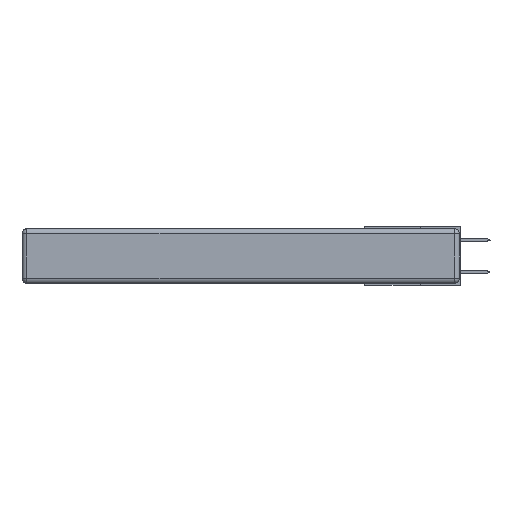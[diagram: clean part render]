
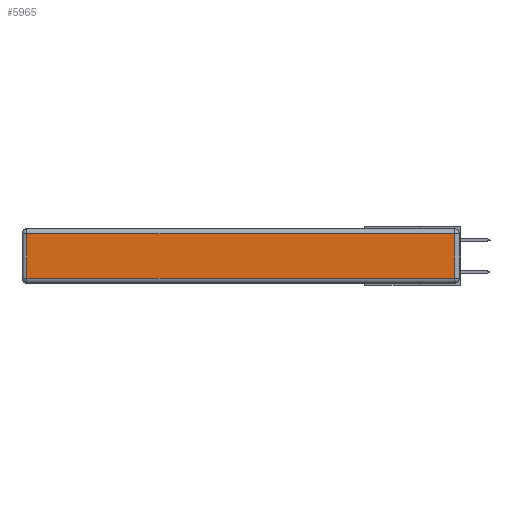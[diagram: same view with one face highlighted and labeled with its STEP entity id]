
A CAD part, left-side view. The second image highlights one B-rep face of the part: STEP entity #5965.
In plain terms, the highlighted planar face has unit normal (-1, 0, 0).
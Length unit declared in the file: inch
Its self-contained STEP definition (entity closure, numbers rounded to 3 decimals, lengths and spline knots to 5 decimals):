
#509 = VECTOR ( 'NONE', #15743, 39.37008 ) ;
#979 = EDGE_LOOP ( 'NONE', ( #4336, #14301, #8746, #16930 ) ) ;
#1898 = CARTESIAN_POINT ( 'NONE',  ( 0., 2.72, -0.03 ) ) ;
#4126 = AXIS2_PLACEMENT_3D ( 'NONE', #28150, #23586, #25646 ) ;
#4127 = EDGE_CURVE ( 'NONE', #7044, #15116, #28561, .T. ) ;
#4336 = ORIENTED_EDGE ( 'NONE', *, *, #13234, .T. ) ;
#5965 = ADVANCED_FACE ( 'NONE', ( #17543 ), #16148, .T. ) ;
#6725 = CARTESIAN_POINT ( 'NONE',  ( 0., 0.03, -0.313 ) ) ;
#7044 = VERTEX_POINT ( 'NONE', #15593 ) ;
#8746 = ORIENTED_EDGE ( 'NONE', *, *, #4127, .T. ) ;
#9346 = EDGE_CURVE ( 'NONE', #16502, #7044, #11460, .T. ) ;
#9361 = DIRECTION ( 'NONE',  ( 0., 0., -1. ) ) ;
#9627 = DIRECTION ( 'NONE',  ( 0., 0., 1. ) ) ;
#11460 = LINE ( 'NONE', #24569, #31768 ) ;
#13234 = EDGE_CURVE ( 'NONE', #30001, #16502, #29903, .T. ) ;
#14301 = ORIENTED_EDGE ( 'NONE', *, *, #9346, .T. ) ;
#15116 = VERTEX_POINT ( 'NONE', #1898 ) ;
#15593 = CARTESIAN_POINT ( 'NONE',  ( 0., 0.03, -0.03 ) ) ;
#15743 = DIRECTION ( 'NONE',  ( 0., 1., 0. ) ) ;
#15960 = CARTESIAN_POINT ( 'NONE',  ( 0., 2.75, -0.03 ) ) ;
#16148 = PLANE ( 'NONE',  #4126 ) ;
#16502 = VERTEX_POINT ( 'NONE', #6725 ) ;
#16624 = VECTOR ( 'NONE', #17464, 39.37008 ) ;
#16930 = ORIENTED_EDGE ( 'NONE', *, *, #19333, .T. ) ;
#17464 = DIRECTION ( 'NONE',  ( 0., -1., 0. ) ) ;
#17543 = FACE_OUTER_BOUND ( 'NONE', #979, .T. ) ;
#19012 = LINE ( 'NONE', #27121, #22499 ) ;
#19333 = EDGE_CURVE ( 'NONE', #15116, #30001, #19012, .T. ) ;
#22499 = VECTOR ( 'NONE', #9361, 39.37008 ) ;
#22830 = CARTESIAN_POINT ( 'NONE',  ( 0., 0., -0.313 ) ) ;
#23586 = DIRECTION ( 'NONE',  ( -1., 0., 0. ) ) ;
#24569 = CARTESIAN_POINT ( 'NONE',  ( 0., 0.03, -0.343 ) ) ;
#25646 = DIRECTION ( 'NONE',  ( 0., 0., 1. ) ) ;
#27121 = CARTESIAN_POINT ( 'NONE',  ( 0., 2.72, -0.343 ) ) ;
#27187 = CARTESIAN_POINT ( 'NONE',  ( 0., 2.72, -0.313 ) ) ;
#28150 = CARTESIAN_POINT ( 'NONE',  ( 0., 0., -0.343 ) ) ;
#28561 = LINE ( 'NONE', #15960, #509 ) ;
#29903 = LINE ( 'NONE', #22830, #16624 ) ;
#30001 = VERTEX_POINT ( 'NONE', #27187 ) ;
#31768 = VECTOR ( 'NONE', #9627, 39.37008 ) ;
